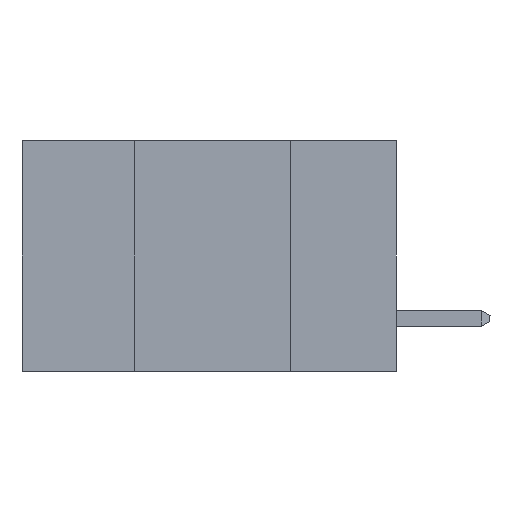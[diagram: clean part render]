
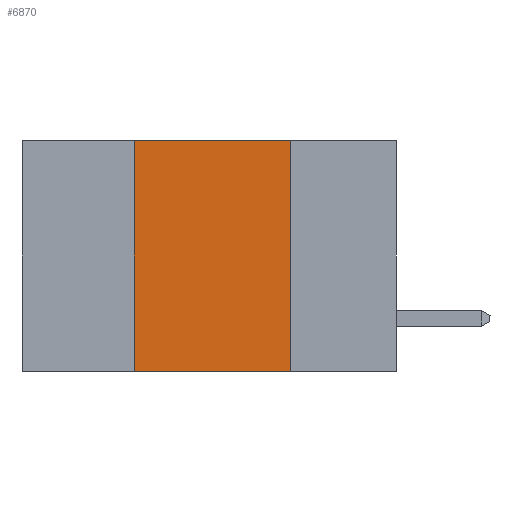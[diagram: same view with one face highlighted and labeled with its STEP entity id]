
A CAD part, left-side view. The second image highlights one B-rep face of the part: STEP entity #6870.
In plain terms, the highlighted planar face has unit normal (-1, 0, 0).
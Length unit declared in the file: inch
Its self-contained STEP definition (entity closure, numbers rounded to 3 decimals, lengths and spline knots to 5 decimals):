
#343 = EDGE_CURVE ( 'NONE', #11606, #3283, #11536, .T. ) ;
#948 = EDGE_CURVE ( 'NONE', #1636, #11606, #11442, .T. ) ;
#1636 = VERTEX_POINT ( 'NONE', #2593 ) ;
#1655 = FACE_OUTER_BOUND ( 'NONE', #7968, .T. ) ;
#1986 = ORIENTED_EDGE ( 'NONE', *, *, #948, .F. ) ;
#2089 = CARTESIAN_POINT ( 'NONE',  ( 0., 0.17, -0.37 ) ) ;
#2448 = PLANE ( 'NONE',  #4345 ) ;
#2459 = ORIENTED_EDGE ( 'NONE', *, *, #9568, .F. ) ;
#2593 = CARTESIAN_POINT ( 'NONE',  ( 0., 0.42, -0.37 ) ) ;
#2618 = DIRECTION ( 'NONE',  ( 0., 0., -1. ) ) ;
#2814 = LINE ( 'NONE', #2089, #10310 ) ;
#3283 = VERTEX_POINT ( 'NONE', #8890 ) ;
#4180 = DIRECTION ( 'NONE',  ( 0., 0., 1. ) ) ;
#4232 = VECTOR ( 'NONE', #4180, 39.37008 ) ;
#4345 = AXIS2_PLACEMENT_3D ( 'NONE', #5142, #6290, #2618 ) ;
#5142 = CARTESIAN_POINT ( 'NONE',  ( 0., 0.6, 0. ) ) ;
#5177 = VERTEX_POINT ( 'NONE', #8892 ) ;
#5461 = LINE ( 'NONE', #10940, #10847 ) ;
#5686 = ORIENTED_EDGE ( 'NONE', *, *, #6015, .T. ) ;
#5709 = ORIENTED_EDGE ( 'NONE', *, *, #343, .F. ) ;
#6015 = EDGE_CURVE ( 'NONE', #1636, #5177, #5461, .T. ) ;
#6254 = DIRECTION ( 'NONE',  ( 0., -1., 0. ) ) ;
#6290 = DIRECTION ( 'NONE',  ( 1., 0., 0. ) ) ;
#6870 = ADVANCED_FACE ( 'NONE', ( #1655 ), #2448, .F. ) ;
#7968 = EDGE_LOOP ( 'NONE', ( #2459, #5709, #1986, #5686 ) ) ;
#8890 = CARTESIAN_POINT ( 'NONE',  ( 0., 0.17, 0. ) ) ;
#8892 = CARTESIAN_POINT ( 'NONE',  ( 0., 0.17, -0.37 ) ) ;
#8904 = VECTOR ( 'NONE', #10649, 39.37008 ) ;
#9472 = CARTESIAN_POINT ( 'NONE',  ( 0., 0.42, 0. ) ) ;
#9568 = EDGE_CURVE ( 'NONE', #3283, #5177, #2814, .T. ) ;
#10310 = VECTOR ( 'NONE', #11166, 39.37008 ) ;
#10649 = DIRECTION ( 'NONE',  ( 0., -1., 0. ) ) ;
#10666 = CARTESIAN_POINT ( 'NONE',  ( 0., 0.42, -0.37 ) ) ;
#10847 = VECTOR ( 'NONE', #6254, 39.37008 ) ;
#10882 = CARTESIAN_POINT ( 'NONE',  ( 0., 0.6, 0. ) ) ;
#10940 = CARTESIAN_POINT ( 'NONE',  ( 0., 0.6, -0.37 ) ) ;
#11166 = DIRECTION ( 'NONE',  ( 0., 0., -1. ) ) ;
#11442 = LINE ( 'NONE', #10666, #4232 ) ;
#11536 = LINE ( 'NONE', #10882, #8904 ) ;
#11606 = VERTEX_POINT ( 'NONE', #9472 ) ;
